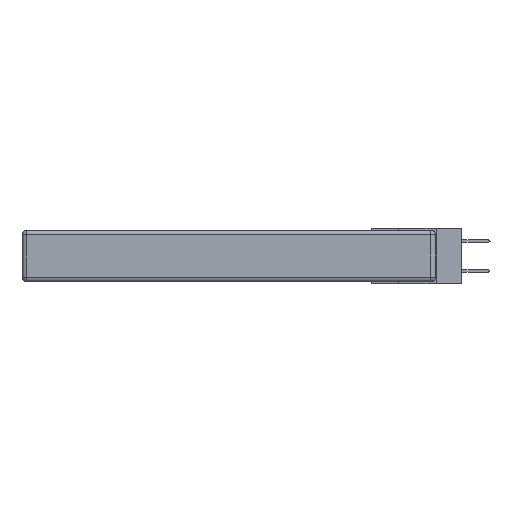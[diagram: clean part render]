
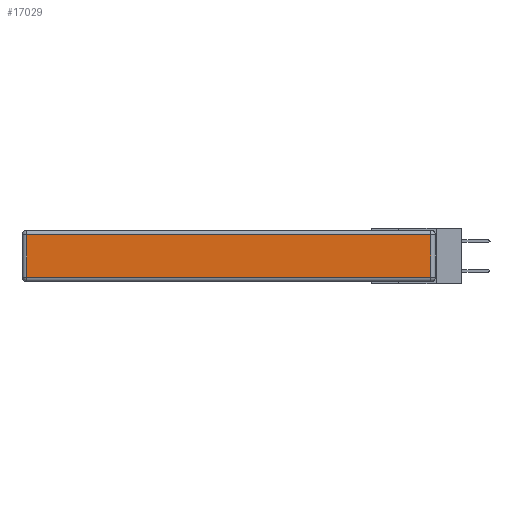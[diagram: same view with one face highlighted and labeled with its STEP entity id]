
A CAD part, left-side view. The second image highlights one B-rep face of the part: STEP entity #17029.
In plain terms, the highlighted planar face has unit normal (-1, 0, 0).
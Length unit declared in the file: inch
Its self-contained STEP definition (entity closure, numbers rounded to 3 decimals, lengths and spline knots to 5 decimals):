
#887 = DIRECTION ( 'NONE',  ( -1., 0., 0. ) ) ;
#1290 = LINE ( 'NONE', #22361, #21419 ) ;
#1570 = VERTEX_POINT ( 'NONE', #22151 ) ;
#2132 = LINE ( 'NONE', #11329, #27352 ) ;
#2194 = DIRECTION ( 'NONE',  ( 0., 1., 0. ) ) ;
#2771 = CARTESIAN_POINT ( 'NONE',  ( 0., 0.03, -0.313 ) ) ;
#2876 = DIRECTION ( 'NONE',  ( 0., -1., 0. ) ) ;
#4814 = DIRECTION ( 'NONE',  ( 0., 0., 1. ) ) ;
#5574 = VERTEX_POINT ( 'NONE', #7636 ) ;
#7600 = PLANE ( 'NONE',  #13398 ) ;
#7636 = CARTESIAN_POINT ( 'NONE',  ( 0., 2.72, -0.313 ) ) ;
#9681 = CARTESIAN_POINT ( 'NONE',  ( 0., 0., -0.313 ) ) ;
#11317 = CARTESIAN_POINT ( 'NONE',  ( 0., 0., -0.343 ) ) ;
#11329 = CARTESIAN_POINT ( 'NONE',  ( 0., 2.75, -0.03 ) ) ;
#12164 = ORIENTED_EDGE ( 'NONE', *, *, #26678, .T. ) ;
#12885 = VECTOR ( 'NONE', #4814, 39.37008 ) ;
#13398 = AXIS2_PLACEMENT_3D ( 'NONE', #11317, #887, #14560 ) ;
#14158 = CARTESIAN_POINT ( 'NONE',  ( 0., 2.72, -0.03 ) ) ;
#14560 = DIRECTION ( 'NONE',  ( 0., 0., 1. ) ) ;
#14857 = LINE ( 'NONE', #25646, #12885 ) ;
#14910 = FACE_OUTER_BOUND ( 'NONE', #20431, .T. ) ;
#15362 = ORIENTED_EDGE ( 'NONE', *, *, #29703, .T. ) ;
#17029 = ADVANCED_FACE ( 'NONE', ( #14910 ), #7600, .T. ) ;
#17757 = DIRECTION ( 'NONE',  ( 0., 0., -1. ) ) ;
#20085 = EDGE_CURVE ( 'NONE', #21286, #1570, #14857, .T. ) ;
#20431 = EDGE_LOOP ( 'NONE', ( #26945, #21791, #12164, #15362 ) ) ;
#21286 = VERTEX_POINT ( 'NONE', #2771 ) ;
#21419 = VECTOR ( 'NONE', #17757, 39.37008 ) ;
#21791 = ORIENTED_EDGE ( 'NONE', *, *, #20085, .T. ) ;
#22151 = CARTESIAN_POINT ( 'NONE',  ( 0., 0.03, -0.03 ) ) ;
#22361 = CARTESIAN_POINT ( 'NONE',  ( 0., 2.72, -0.343 ) ) ;
#22867 = LINE ( 'NONE', #9681, #28592 ) ;
#25646 = CARTESIAN_POINT ( 'NONE',  ( 0., 0.03, -0.343 ) ) ;
#26678 = EDGE_CURVE ( 'NONE', #1570, #26779, #2132, .T. ) ;
#26779 = VERTEX_POINT ( 'NONE', #14158 ) ;
#26945 = ORIENTED_EDGE ( 'NONE', *, *, #29522, .T. ) ;
#27352 = VECTOR ( 'NONE', #2194, 39.37008 ) ;
#28592 = VECTOR ( 'NONE', #2876, 39.37008 ) ;
#29522 = EDGE_CURVE ( 'NONE', #5574, #21286, #22867, .T. ) ;
#29703 = EDGE_CURVE ( 'NONE', #26779, #5574, #1290, .T. ) ;
